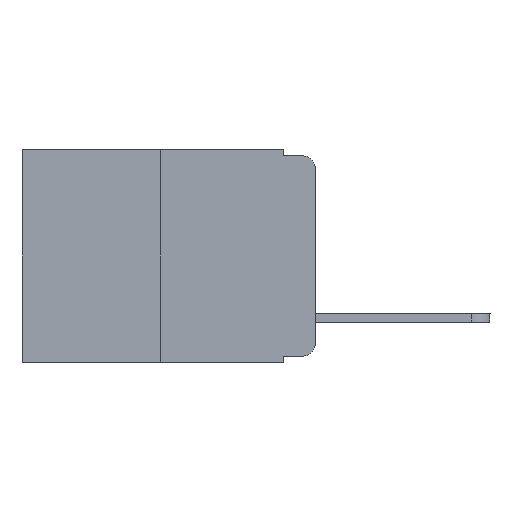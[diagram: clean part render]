
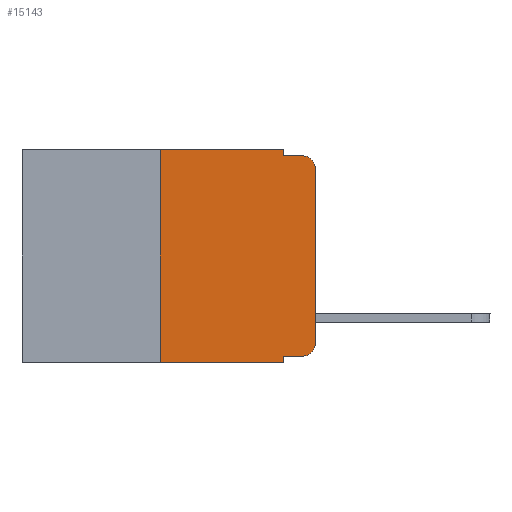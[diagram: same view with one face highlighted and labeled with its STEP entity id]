
A CAD part, left-side view. The second image highlights one B-rep face of the part: STEP entity #15143.
In plain terms, the highlighted planar face has unit normal (-1, 0, 0).
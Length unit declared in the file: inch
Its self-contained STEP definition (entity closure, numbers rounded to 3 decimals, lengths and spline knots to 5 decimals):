
#545 = LINE ( 'NONE', #13372, #13691 ) ;
#694 = CARTESIAN_POINT ( 'NONE',  ( 0., 0.473, 0. ) ) ;
#799 = LINE ( 'NONE', #17533, #10196 ) ;
#854 = LINE ( 'NONE', #2328, #15132 ) ;
#874 = DIRECTION ( 'NONE',  ( 1., 0., 0. ) ) ;
#931 = VERTEX_POINT ( 'NONE', #4135 ) ;
#1922 = ORIENTED_EDGE ( 'NONE', *, *, #5190, .F. ) ;
#2055 = DIRECTION ( 'NONE',  ( -1., 0., 0. ) ) ;
#2094 = EDGE_CURVE ( 'NONE', #16846, #2462, #545, .T. ) ;
#2316 = ORIENTED_EDGE ( 'NONE', *, *, #6601, .F. ) ;
#2328 = CARTESIAN_POINT ( 'NONE',  ( 0., 0.473, -0.343 ) ) ;
#2462 = VERTEX_POINT ( 'NONE', #9237 ) ;
#2982 = EDGE_CURVE ( 'NONE', #10397, #4822, #854, .T. ) ;
#3263 = EDGE_CURVE ( 'NONE', #17562, #15189, #10415, .T. ) ;
#3269 = DIRECTION ( 'NONE',  ( 0., 0., -1. ) ) ;
#3484 = ORIENTED_EDGE ( 'NONE', *, *, #16576, .F. ) ;
#3485 = PLANE ( 'NONE',  #14697 ) ;
#3582 = CARTESIAN_POINT ( 'NONE',  ( 0., 0.051, -0.01 ) ) ;
#3749 = DIRECTION ( 'NONE',  ( 0., 0., -1. ) ) ;
#4135 = CARTESIAN_POINT ( 'NONE',  ( 0., 0.25, 0. ) ) ;
#4364 = AXIS2_PLACEMENT_3D ( 'NONE', #12736, #14034, #11253 ) ;
#4663 = CARTESIAN_POINT ( 'NONE',  ( 0., 0.051, -0.01 ) ) ;
#4822 = VERTEX_POINT ( 'NONE', #5517 ) ;
#5190 = EDGE_CURVE ( 'NONE', #931, #15757, #14154, .T. ) ;
#5378 = VECTOR ( 'NONE', #12477, 39.37008 ) ;
#5517 = CARTESIAN_POINT ( 'NONE',  ( 0., 0.051, -0.343 ) ) ;
#5587 = CARTESIAN_POINT ( 'NONE',  ( 0., 0.25, -0.343 ) ) ;
#6154 = EDGE_CURVE ( 'NONE', #10397, #931, #12871, .T. ) ;
#6159 = ORIENTED_EDGE ( 'NONE', *, *, #6154, .F. ) ;
#6361 = CIRCLE ( 'NONE', #15875, 0.02 ) ;
#6458 = CARTESIAN_POINT ( 'NONE',  ( 0., 0.02, -0.333 ) ) ;
#6601 = EDGE_CURVE ( 'NONE', #17562, #4822, #16663, .T. ) ;
#6720 = ORIENTED_EDGE ( 'NONE', *, *, #3263, .T. ) ;
#6990 = DIRECTION ( 'NONE',  ( 0., -1., 0. ) ) ;
#7019 = VECTOR ( 'NONE', #10343, 39.37008 ) ;
#7755 = FACE_OUTER_BOUND ( 'NONE', #15016, .T. ) ;
#8245 = EDGE_CURVE ( 'NONE', #15189, #16846, #11204, .T. ) ;
#8297 = VECTOR ( 'NONE', #17909, 39.37008 ) ;
#8584 = CARTESIAN_POINT ( 'NONE',  ( 0., 0.25, 0. ) ) ;
#9043 = VECTOR ( 'NONE', #10863, 39.37008 ) ;
#9237 = CARTESIAN_POINT ( 'NONE',  ( 0., 0., -0.03 ) ) ;
#9346 = DIRECTION ( 'NONE',  ( 0., 0., -1. ) ) ;
#9811 = ORIENTED_EDGE ( 'NONE', *, *, #2982, .T. ) ;
#10196 = VECTOR ( 'NONE', #9346, 39.37008 ) ;
#10343 = DIRECTION ( 'NONE',  ( 0., -1., 0. ) ) ;
#10397 = VERTEX_POINT ( 'NONE', #5587 ) ;
#10415 = LINE ( 'NONE', #16524, #8297 ) ;
#10863 = DIRECTION ( 'NONE',  ( 0., 0., 1. ) ) ;
#11112 = CARTESIAN_POINT ( 'NONE',  ( 0., 0.02, -0.01 ) ) ;
#11204 = CIRCLE ( 'NONE', #4364, 0.02 ) ;
#11253 = DIRECTION ( 'NONE',  ( 0., 0., -1. ) ) ;
#11502 = VERTEX_POINT ( 'NONE', #3582 ) ;
#11673 = VERTEX_POINT ( 'NONE', #11112 ) ;
#11704 = VECTOR ( 'NONE', #6990, 39.37008 ) ;
#11772 = ORIENTED_EDGE ( 'NONE', *, *, #2094, .T. ) ;
#12199 = DIRECTION ( 'NONE',  ( 0., -1., 0. ) ) ;
#12477 = DIRECTION ( 'NONE',  ( 0., 0., -1. ) ) ;
#12736 = CARTESIAN_POINT ( 'NONE',  ( 0., 0.02, -0.313 ) ) ;
#12871 = LINE ( 'NONE', #8584, #9043 ) ;
#13084 = ORIENTED_EDGE ( 'NONE', *, *, #8245, .T. ) ;
#13372 = CARTESIAN_POINT ( 'NONE',  ( 0., 0., 0. ) ) ;
#13539 = CARTESIAN_POINT ( 'NONE',  ( 0., 0., -0.313 ) ) ;
#13691 = VECTOR ( 'NONE', #17821, 39.37008 ) ;
#13774 = CARTESIAN_POINT ( 'NONE',  ( 0., 0.051, 0. ) ) ;
#13874 = CARTESIAN_POINT ( 'NONE',  ( 0., 0.051, 0. ) ) ;
#14034 = DIRECTION ( 'NONE',  ( -1., 0., 0. ) ) ;
#14154 = LINE ( 'NONE', #15543, #11704 ) ;
#14325 = CARTESIAN_POINT ( 'NONE',  ( 0., 0.051, -0.333 ) ) ;
#14337 = EDGE_CURVE ( 'NONE', #2462, #11673, #6361, .T. ) ;
#14531 = LINE ( 'NONE', #4663, #7019 ) ;
#14697 = AXIS2_PLACEMENT_3D ( 'NONE', #694, #874, #3749 ) ;
#15016 = EDGE_LOOP ( 'NONE', ( #11772, #17341, #3484, #16651, #1922, #6159, #9811, #2316, #6720, #13084 ) ) ;
#15132 = VECTOR ( 'NONE', #12199, 39.37008 ) ;
#15143 = ADVANCED_FACE ( 'NONE', ( #7755 ), #3485, .F. ) ;
#15189 = VERTEX_POINT ( 'NONE', #6458 ) ;
#15543 = CARTESIAN_POINT ( 'NONE',  ( 0., 0.473, 0. ) ) ;
#15757 = VERTEX_POINT ( 'NONE', #13774 ) ;
#15875 = AXIS2_PLACEMENT_3D ( 'NONE', #17772, #2055, #3269 ) ;
#16524 = CARTESIAN_POINT ( 'NONE',  ( 0., 0.051, -0.333 ) ) ;
#16576 = EDGE_CURVE ( 'NONE', #11502, #11673, #14531, .T. ) ;
#16651 = ORIENTED_EDGE ( 'NONE', *, *, #18129, .F. ) ;
#16663 = LINE ( 'NONE', #13874, #5378 ) ;
#16846 = VERTEX_POINT ( 'NONE', #13539 ) ;
#17341 = ORIENTED_EDGE ( 'NONE', *, *, #14337, .T. ) ;
#17533 = CARTESIAN_POINT ( 'NONE',  ( 0., 0.051, 0. ) ) ;
#17562 = VERTEX_POINT ( 'NONE', #14325 ) ;
#17772 = CARTESIAN_POINT ( 'NONE',  ( 0., 0.02, -0.03 ) ) ;
#17821 = DIRECTION ( 'NONE',  ( 0., 0., 1. ) ) ;
#17909 = DIRECTION ( 'NONE',  ( 0., -1., 0. ) ) ;
#18129 = EDGE_CURVE ( 'NONE', #15757, #11502, #799, .T. ) ;
